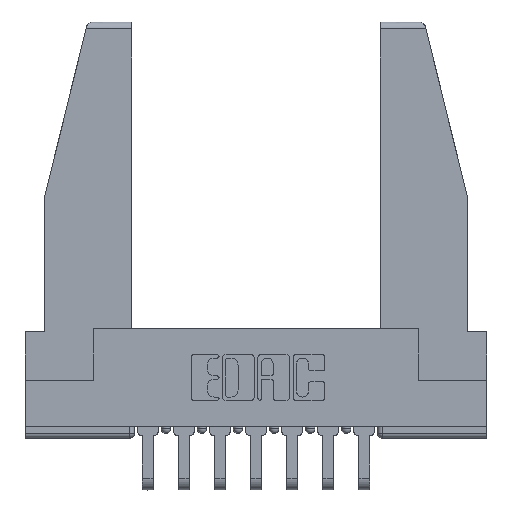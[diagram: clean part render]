
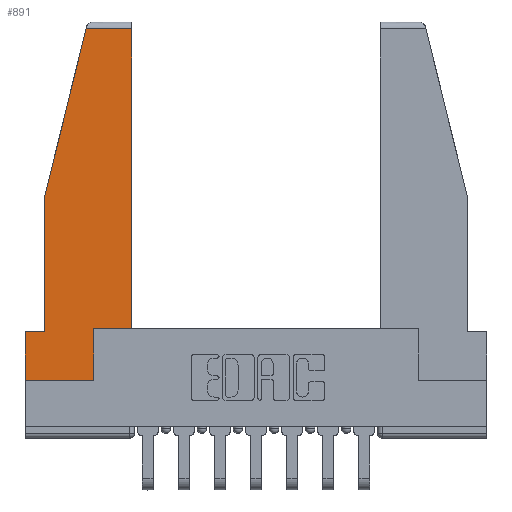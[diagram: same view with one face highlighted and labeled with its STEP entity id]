
A CAD part, top view. The second image highlights one B-rep face of the part: STEP entity #891.
In plain terms, the highlighted planar face has unit normal (0, 0, 1).
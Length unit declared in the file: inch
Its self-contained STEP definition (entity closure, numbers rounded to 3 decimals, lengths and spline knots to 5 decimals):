
#349 = CARTESIAN_POINT ( 'NONE',  ( 0., 0., 0. ) ) ;
#733 = ORIENTED_EDGE ( 'NONE', *, *, #2947, .T. ) ;
#891 = ADVANCED_FACE ( 'NONE', ( #10674 ), #1676, .T. ) ;
#1194 = CARTESIAN_POINT ( 'NONE',  ( 0.461, 0.223, 0. ) ) ;
#1303 = DIRECTION ( 'NONE',  ( -0.239, -0.971, 0. ) ) ;
#1384 = CARTESIAN_POINT ( 'NONE',  ( 0.271, 1.55, 0. ) ) ;
#1534 = CARTESIAN_POINT ( 'NONE',  ( 0.086, 0.8, 0. ) ) ;
#1584 = EDGE_CURVE ( 'NONE', #4894, #11338, #8572, .T. ) ;
#1676 = PLANE ( 'NONE',  #2456 ) ;
#2172 = VERTEX_POINT ( 'NONE', #1194 ) ;
#2319 = CARTESIAN_POINT ( 'NONE',  ( 0., 0.21, 0. ) ) ;
#2376 = CARTESIAN_POINT ( 'NONE',  ( 0.461, 1.52, 0. ) ) ;
#2456 = AXIS2_PLACEMENT_3D ( 'NONE', #3960, #14043, #4254 ) ;
#2947 = EDGE_CURVE ( 'NONE', #3792, #4894, #10221, .T. ) ;
#3075 = LINE ( 'NONE', #5414, #9827 ) ;
#3148 = DIRECTION ( 'NONE',  ( 0., -1., 0. ) ) ;
#3400 = VECTOR ( 'NONE', #6770, 39.37008 ) ;
#3436 = DIRECTION ( 'NONE',  ( 1., 0., 0. ) ) ;
#3448 = ORIENTED_EDGE ( 'NONE', *, *, #1584, .T. ) ;
#3471 = VERTEX_POINT ( 'NONE', #2376 ) ;
#3792 = VERTEX_POINT ( 'NONE', #6836 ) ;
#3817 = LINE ( 'NONE', #1384, #6602 ) ;
#3923 = CARTESIAN_POINT ( 'NONE',  ( 0., 0.21, 0. ) ) ;
#3960 = CARTESIAN_POINT ( 'NONE',  ( 0., 0., 0. ) ) ;
#4254 = DIRECTION ( 'NONE',  ( 1., 0., 0. ) ) ;
#4510 = LINE ( 'NONE', #5750, #6144 ) ;
#4680 = EDGE_CURVE ( 'NONE', #2172, #3471, #6598, .T. ) ;
#4786 = CARTESIAN_POINT ( 'NONE',  ( 0.297, 0., 0. ) ) ;
#4790 = ORIENTED_EDGE ( 'NONE', *, *, #10680, .T. ) ;
#4894 = VERTEX_POINT ( 'NONE', #3923 ) ;
#5104 = EDGE_CURVE ( 'NONE', #3471, #13843, #9023, .T. ) ;
#5261 = VECTOR ( 'NONE', #14182, 39.37008 ) ;
#5414 = CARTESIAN_POINT ( 'NONE',  ( 0.086, 0.8, 0. ) ) ;
#5750 = CARTESIAN_POINT ( 'NONE',  ( 0.297, 0., 0. ) ) ;
#6144 = VECTOR ( 'NONE', #7870, 39.37008 ) ;
#6314 = VECTOR ( 'NONE', #6928, 39.37008 ) ;
#6526 = VERTEX_POINT ( 'NONE', #14170 ) ;
#6598 = LINE ( 'NONE', #11102, #11545 ) ;
#6602 = VECTOR ( 'NONE', #1303, 39.37008 ) ;
#6770 = DIRECTION ( 'NONE',  ( -1., 0., 0. ) ) ;
#6836 = CARTESIAN_POINT ( 'NONE',  ( 0.086, 0.21, 0. ) ) ;
#6907 = CARTESIAN_POINT ( 'NONE',  ( 0., 1.52, 0. ) ) ;
#6928 = DIRECTION ( 'NONE',  ( 1., 0., 0. ) ) ;
#7217 = ORIENTED_EDGE ( 'NONE', *, *, #9366, .T. ) ;
#7238 = VERTEX_POINT ( 'NONE', #4786 ) ;
#7247 = VECTOR ( 'NONE', #11168, 39.37008 ) ;
#7749 = LINE ( 'NONE', #7883, #6314 ) ;
#7870 = DIRECTION ( 'NONE',  ( 0., 1., 0. ) ) ;
#7883 = CARTESIAN_POINT ( 'NONE',  ( 0.297, 0.223, 0. ) ) ;
#8572 = LINE ( 'NONE', #9734, #5261 ) ;
#8789 = DIRECTION ( 'NONE',  ( 0., 1., 0. ) ) ;
#8843 = VECTOR ( 'NONE', #3436, 39.37008 ) ;
#9023 = LINE ( 'NONE', #6907, #3400 ) ;
#9218 = ORIENTED_EDGE ( 'NONE', *, *, #4680, .T. ) ;
#9366 = EDGE_CURVE ( 'NONE', #11338, #7238, #13607, .T. ) ;
#9734 = CARTESIAN_POINT ( 'NONE',  ( 0., 0.21, 0. ) ) ;
#9827 = VECTOR ( 'NONE', #3148, 39.37008 ) ;
#10221 = LINE ( 'NONE', #2319, #7247 ) ;
#10674 = FACE_OUTER_BOUND ( 'NONE', #13233, .T. ) ;
#10680 = EDGE_CURVE ( 'NONE', #6526, #2172, #7749, .T. ) ;
#11102 = CARTESIAN_POINT ( 'NONE',  ( 0.461, 0.223, 0. ) ) ;
#11168 = DIRECTION ( 'NONE',  ( -1., 0., 0. ) ) ;
#11236 = VERTEX_POINT ( 'NONE', #1534 ) ;
#11338 = VERTEX_POINT ( 'NONE', #12131 ) ;
#11545 = VECTOR ( 'NONE', #8789, 39.37008 ) ;
#11870 = EDGE_CURVE ( 'NONE', #11236, #3792, #3075, .T. ) ;
#11921 = ORIENTED_EDGE ( 'NONE', *, *, #11870, .T. ) ;
#12131 = CARTESIAN_POINT ( 'NONE',  ( 0., 0., 0. ) ) ;
#12827 = CARTESIAN_POINT ( 'NONE',  ( 0.2636, 1.52, 0. ) ) ;
#13054 = ORIENTED_EDGE ( 'NONE', *, *, #5104, .T. ) ;
#13233 = EDGE_LOOP ( 'NONE', ( #9218, #13054, #13647, #11921, #733, #3448, #7217, #14221, #4790 ) ) ;
#13607 = LINE ( 'NONE', #349, #8843 ) ;
#13647 = ORIENTED_EDGE ( 'NONE', *, *, #14294, .T. ) ;
#13767 = EDGE_CURVE ( 'NONE', #7238, #6526, #4510, .T. ) ;
#13843 = VERTEX_POINT ( 'NONE', #12827 ) ;
#14043 = DIRECTION ( 'NONE',  ( 0., 0., 1. ) ) ;
#14170 = CARTESIAN_POINT ( 'NONE',  ( 0.297, 0.223, 0. ) ) ;
#14182 = DIRECTION ( 'NONE',  ( 0., -1., 0. ) ) ;
#14221 = ORIENTED_EDGE ( 'NONE', *, *, #13767, .T. ) ;
#14294 = EDGE_CURVE ( 'NONE', #13843, #11236, #3817, .T. ) ;
